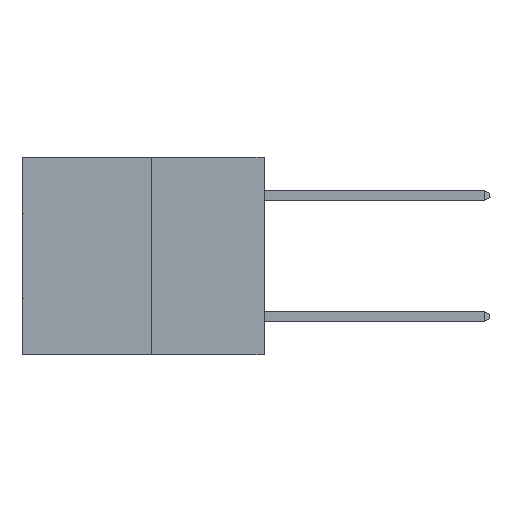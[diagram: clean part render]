
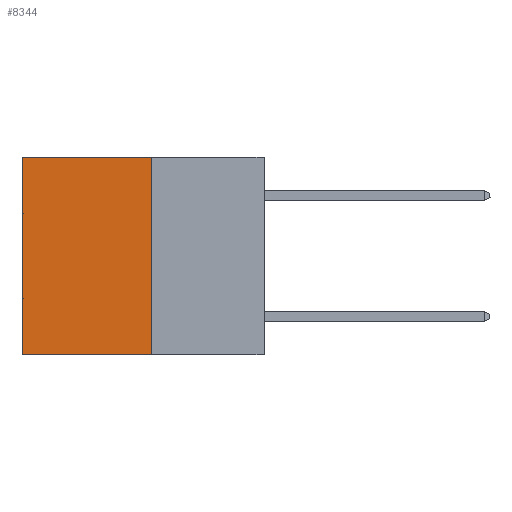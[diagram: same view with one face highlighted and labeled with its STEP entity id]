
A CAD part, left-side view. The second image highlights one B-rep face of the part: STEP entity #8344.
In plain terms, the highlighted planar face has unit normal (-1, 0, 0).
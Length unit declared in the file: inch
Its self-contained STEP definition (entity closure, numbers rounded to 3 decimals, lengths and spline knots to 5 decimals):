
#237 = ORIENTED_EDGE ( 'NONE', *, *, #23870, .T. ) ;
#293 = EDGE_CURVE ( 'NONE', #32654, #19238, #31112, .T. ) ;
#1536 = CARTESIAN_POINT ( 'NONE',  ( 0.3165, 0.6, -0.49 ) ) ;
#5112 = PLANE ( 'NONE',  #18321 ) ;
#8344 = ADVANCED_FACE ( 'NONE', ( #29735 ), #5112, .F. ) ;
#8933 = CARTESIAN_POINT ( 'NONE',  ( 0.3165, 0.28, 0. ) ) ;
#10172 = VERTEX_POINT ( 'NONE', #1536 ) ;
#10602 = VERTEX_POINT ( 'NONE', #32810 ) ;
#10706 = VECTOR ( 'NONE', #19741, 39.37008 ) ;
#10903 = LINE ( 'NONE', #31213, #23087 ) ;
#13429 = ORIENTED_EDGE ( 'NONE', *, *, #21720, .F. ) ;
#14950 = DIRECTION ( 'NONE',  ( 0., 1., 0. ) ) ;
#16634 = ORIENTED_EDGE ( 'NONE', *, *, #293, .T. ) ;
#17472 = CARTESIAN_POINT ( 'NONE',  ( 0.3165, 0.28, -0.49 ) ) ;
#18321 = AXIS2_PLACEMENT_3D ( 'NONE', #18633, #27180, #25672 ) ;
#18633 = CARTESIAN_POINT ( 'NONE',  ( 0.3165, 0.28, -0.49 ) ) ;
#18862 = DIRECTION ( 'NONE',  ( 0., 0., -1. ) ) ;
#19238 = VERTEX_POINT ( 'NONE', #24445 ) ;
#19741 = DIRECTION ( 'NONE',  ( 0., 1., 0. ) ) ;
#21163 = LINE ( 'NONE', #26856, #21579 ) ;
#21579 = VECTOR ( 'NONE', #18862, 39.37008 ) ;
#21720 = EDGE_CURVE ( 'NONE', #10602, #10172, #26286, .T. ) ;
#22632 = CARTESIAN_POINT ( 'NONE',  ( 0.3165, 0.28, 0. ) ) ;
#23087 = VECTOR ( 'NONE', #33728, 39.37008 ) ;
#23870 = EDGE_CURVE ( 'NONE', #19238, #10172, #21163, .T. ) ;
#24445 = CARTESIAN_POINT ( 'NONE',  ( 0.3165, 0.6, 0. ) ) ;
#25672 = DIRECTION ( 'NONE',  ( 0., 0., -1. ) ) ;
#26286 = LINE ( 'NONE', #17472, #29139 ) ;
#26856 = CARTESIAN_POINT ( 'NONE',  ( 0.3165, 0.6, -0.49 ) ) ;
#27180 = DIRECTION ( 'NONE',  ( 1., 0., 0. ) ) ;
#29139 = VECTOR ( 'NONE', #14950, 39.37008 ) ;
#29735 = FACE_OUTER_BOUND ( 'NONE', #30267, .T. ) ;
#30267 = EDGE_LOOP ( 'NONE', ( #237, #13429, #33326, #16634 ) ) ;
#31112 = LINE ( 'NONE', #8933, #10706 ) ;
#31213 = CARTESIAN_POINT ( 'NONE',  ( 0.3165, 0.28, -0.49 ) ) ;
#32654 = VERTEX_POINT ( 'NONE', #22632 ) ;
#32810 = CARTESIAN_POINT ( 'NONE',  ( 0.3165, 0.28, -0.49 ) ) ;
#32838 = EDGE_CURVE ( 'NONE', #32654, #10602, #10903, .T. ) ;
#33326 = ORIENTED_EDGE ( 'NONE', *, *, #32838, .F. ) ;
#33728 = DIRECTION ( 'NONE',  ( 0., 0., -1. ) ) ;
